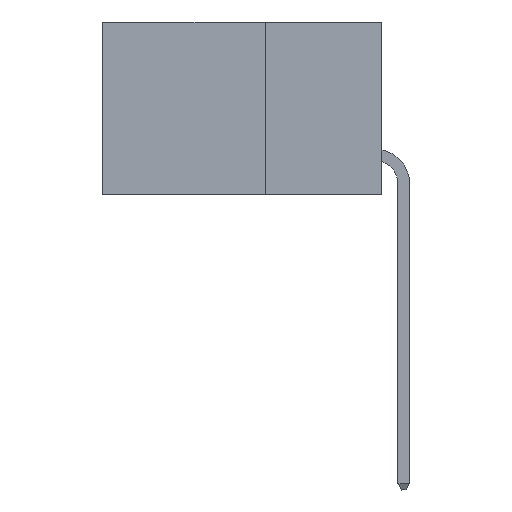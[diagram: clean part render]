
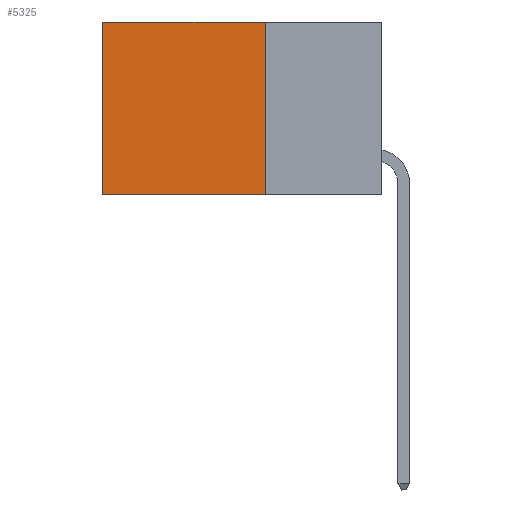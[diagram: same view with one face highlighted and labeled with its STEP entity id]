
A CAD part, left-side view. The second image highlights one B-rep face of the part: STEP entity #5325.
In plain terms, the highlighted planar face has unit normal (-1, 0, 0).
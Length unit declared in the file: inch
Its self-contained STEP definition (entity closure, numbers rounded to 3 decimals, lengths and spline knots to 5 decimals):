
#1812 = VECTOR ( 'NONE', #35575, 39.37008 ) ;
#4440 = DIRECTION ( 'NONE',  ( 1., 0., 0. ) ) ;
#5070 = DIRECTION ( 'NONE',  ( 0., 0., -1. ) ) ;
#5325 = ADVANCED_FACE ( 'NONE', ( #38785 ), #27153, .F. ) ;
#6835 = VERTEX_POINT ( 'NONE', #14542 ) ;
#8398 = ORIENTED_EDGE ( 'NONE', *, *, #16038, .T. ) ;
#8601 = EDGE_CURVE ( 'NONE', #42333, #6835, #25719, .T. ) ;
#8685 = ORIENTED_EDGE ( 'NONE', *, *, #8601, .F. ) ;
#12070 = ORIENTED_EDGE ( 'NONE', *, *, #19522, .T. ) ;
#12164 = CARTESIAN_POINT ( 'NONE',  ( 0.2875, 0.6, 0. ) ) ;
#14542 = CARTESIAN_POINT ( 'NONE',  ( 0.2875, 0.6, -0.37 ) ) ;
#16038 = EDGE_CURVE ( 'NONE', #28283, #27876, #38148, .T. ) ;
#18888 = VECTOR ( 'NONE', #19948, 39.37008 ) ;
#19522 = EDGE_CURVE ( 'NONE', #27876, #6835, #40061, .T. ) ;
#19793 = CARTESIAN_POINT ( 'NONE',  ( 0.2875, 0.6, 0. ) ) ;
#19948 = DIRECTION ( 'NONE',  ( 0., 0., -1. ) ) ;
#25104 = CARTESIAN_POINT ( 'NONE',  ( 0.2875, 0.25, 0. ) ) ;
#25719 = LINE ( 'NONE', #28616, #45147 ) ;
#26155 = CARTESIAN_POINT ( 'NONE',  ( 0.2875, 0.25, 0. ) ) ;
#27153 = PLANE ( 'NONE',  #27323 ) ;
#27323 = AXIS2_PLACEMENT_3D ( 'NONE', #25104, #4440, #5070 ) ;
#27876 = VERTEX_POINT ( 'NONE', #12164 ) ;
#28283 = VERTEX_POINT ( 'NONE', #26155 ) ;
#28616 = CARTESIAN_POINT ( 'NONE',  ( 0.2875, 0.25, -0.37 ) ) ;
#29007 = EDGE_CURVE ( 'NONE', #28283, #42333, #30343, .T. ) ;
#30343 = LINE ( 'NONE', #35725, #1812 ) ;
#30356 = DIRECTION ( 'NONE',  ( 0., 1., 0. ) ) ;
#31439 = VECTOR ( 'NONE', #30356, 39.37008 ) ;
#35575 = DIRECTION ( 'NONE',  ( 0., 0., -1. ) ) ;
#35720 = EDGE_LOOP ( 'NONE', ( #12070, #8685, #45472, #8398 ) ) ;
#35725 = CARTESIAN_POINT ( 'NONE',  ( 0.2875, 0.25, 0. ) ) ;
#38148 = LINE ( 'NONE', #49001, #31439 ) ;
#38785 = FACE_OUTER_BOUND ( 'NONE', #35720, .T. ) ;
#40061 = LINE ( 'NONE', #19793, #18888 ) ;
#40336 = DIRECTION ( 'NONE',  ( 0., 1., 0. ) ) ;
#40651 = CARTESIAN_POINT ( 'NONE',  ( 0.2875, 0.25, -0.37 ) ) ;
#42333 = VERTEX_POINT ( 'NONE', #40651 ) ;
#45147 = VECTOR ( 'NONE', #40336, 39.37008 ) ;
#45472 = ORIENTED_EDGE ( 'NONE', *, *, #29007, .F. ) ;
#49001 = CARTESIAN_POINT ( 'NONE',  ( 0.2875, 0.25, 0. ) ) ;
